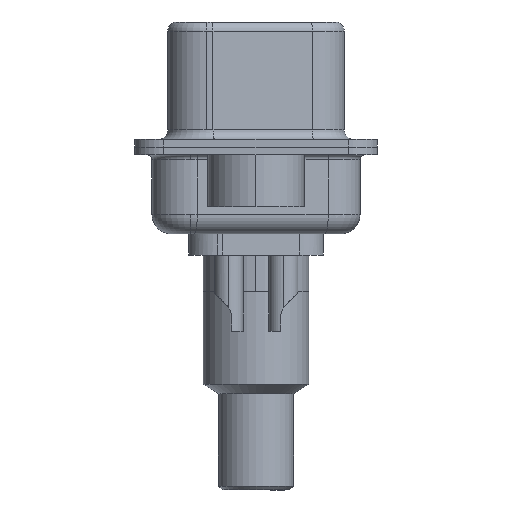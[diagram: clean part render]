
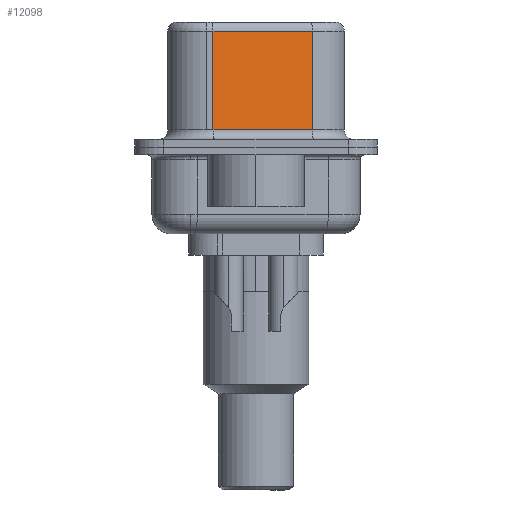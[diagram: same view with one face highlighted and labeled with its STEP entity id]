
A CAD part, left-side view. The second image highlights one B-rep face of the part: STEP entity #12098.
In plain terms, the highlighted planar face has unit normal (-0.985, -0.174, 0).
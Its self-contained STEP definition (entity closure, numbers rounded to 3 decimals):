
#361 = AXIS2_PLACEMENT_3D ( 'NONE', #14623, #9950, #502 ) ;
#502 = DIRECTION ( 'NONE',  ( -0.174, 0.985, 0. ) ) ;
#1468 = ORIENTED_EDGE ( 'NONE', *, *, #10772, .T. ) ;
#2514 = LINE ( 'NONE', #8028, #9921 ) ;
#2741 = ORIENTED_EDGE ( 'NONE', *, *, #16155, .T. ) ;
#2960 = CARTESIAN_POINT ( 'NONE',  ( 3.655, 2.233, 0.9 ) ) ;
#4213 = DIRECTION ( 'NONE',  ( -0.174, 0.985, 0. ) ) ;
#4656 = ORIENTED_EDGE ( 'NONE', *, *, #6862, .T. ) ;
#4756 = VERTEX_POINT ( 'NONE', #19456 ) ;
#5193 = VERTEX_POINT ( 'NONE', #2960 ) ;
#5517 = CARTESIAN_POINT ( 'NONE',  ( 3.655, 2.233, 6.02 ) ) ;
#5915 = EDGE_LOOP ( 'NONE', ( #7888, #4656, #1468, #2741 ) ) ;
#6862 = EDGE_CURVE ( 'NONE', #13573, #9352, #18539, .T. ) ;
#7276 = LINE ( 'NONE', #19623, #15671 ) ;
#7385 = FACE_OUTER_BOUND ( 'NONE', #5915, .T. ) ;
#7888 = ORIENTED_EDGE ( 'NONE', *, *, #8774, .F. ) ;
#8028 = CARTESIAN_POINT ( 'NONE',  ( 3.655, 2.233, 6.52 ) ) ;
#8774 = EDGE_CURVE ( 'NONE', #13573, #4756, #14409, .T. ) ;
#9352 = VERTEX_POINT ( 'NONE', #5517 ) ;
#9921 = VECTOR ( 'NONE', #11128, 1000. ) ;
#9950 = DIRECTION ( 'NONE',  ( 0.985, 0.174, 0. ) ) ;
#10141 = DIRECTION ( 'NONE',  ( 0.174, -0.985, 0. ) ) ;
#10772 = EDGE_CURVE ( 'NONE', #9352, #5193, #2514, .T. ) ;
#11128 = DIRECTION ( 'NONE',  ( 0., 0., -1. ) ) ;
#11167 = CARTESIAN_POINT ( 'NONE',  ( 4.565, -2.927, 6.52 ) ) ;
#11533 = DIRECTION ( 'NONE',  ( 0., 0., -1. ) ) ;
#12098 = ADVANCED_FACE ( 'NONE', ( #7385 ), #19427, .F. ) ;
#13573 = VERTEX_POINT ( 'NONE', #18057 ) ;
#13935 = VECTOR ( 'NONE', #11533, 1000. ) ;
#14409 = LINE ( 'NONE', #11167, #13935 ) ;
#14623 = CARTESIAN_POINT ( 'NONE',  ( 4.565, -2.927, 6.52 ) ) ;
#15671 = VECTOR ( 'NONE', #10141, 1000. ) ;
#16155 = EDGE_CURVE ( 'NONE', #5193, #4756, #7276, .T. ) ;
#18025 = VECTOR ( 'NONE', #4213, 1000. ) ;
#18057 = CARTESIAN_POINT ( 'NONE',  ( 4.565, -2.927, 6.02 ) ) ;
#18539 = LINE ( 'NONE', #19542, #18025 ) ;
#19427 = PLANE ( 'NONE',  #361 ) ;
#19456 = CARTESIAN_POINT ( 'NONE',  ( 4.565, -2.927, 0.9 ) ) ;
#19542 = CARTESIAN_POINT ( 'NONE',  ( 4.565, -2.927, 6.02 ) ) ;
#19623 = CARTESIAN_POINT ( 'NONE',  ( 4.565, -2.927, 0.9 ) ) ;
